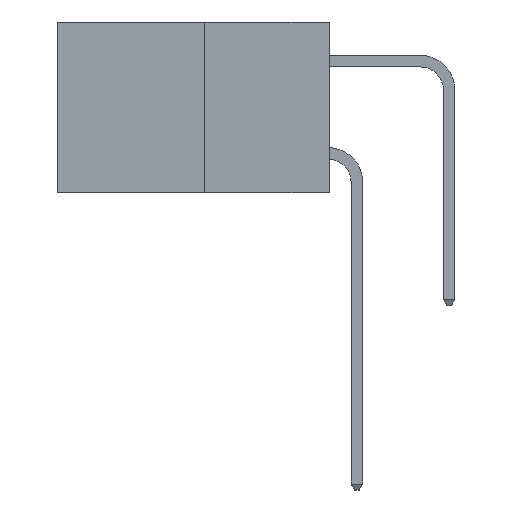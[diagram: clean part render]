
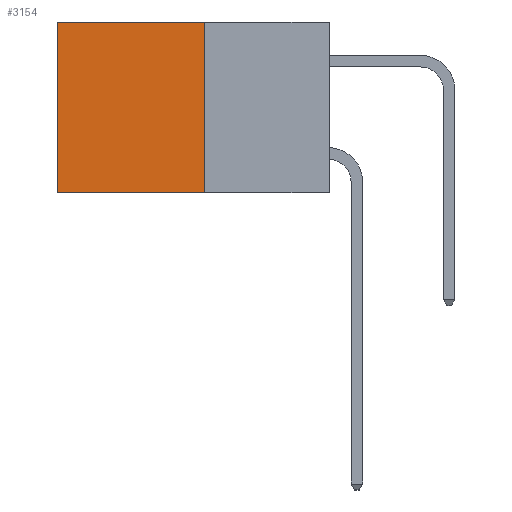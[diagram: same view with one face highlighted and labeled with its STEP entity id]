
A CAD part, left-side view. The second image highlights one B-rep face of the part: STEP entity #3154.
In plain terms, the highlighted planar face has unit normal (-1, 0, 0).
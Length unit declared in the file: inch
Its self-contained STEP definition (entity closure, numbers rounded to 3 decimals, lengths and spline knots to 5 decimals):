
#907 = EDGE_CURVE ( 'NONE', #5176, #29752, #3105, .T. ) ;
#1414 = EDGE_LOOP ( 'NONE', ( #25171, #21873, #22550, #12734 ) ) ;
#3019 = CARTESIAN_POINT ( 'NONE',  ( 0.277, 0.27, -0.37 ) ) ;
#3105 = LINE ( 'NONE', #26412, #15734 ) ;
#3154 = ADVANCED_FACE ( 'NONE', ( #15588 ), #24416, .F. ) ;
#4847 = VERTEX_POINT ( 'NONE', #13931 ) ;
#5176 = VERTEX_POINT ( 'NONE', #19872 ) ;
#7622 = VERTEX_POINT ( 'NONE', #25596 ) ;
#8562 = VECTOR ( 'NONE', #15060, 39.37008 ) ;
#9820 = DIRECTION ( 'NONE',  ( 0., 1., 0. ) ) ;
#10041 = DIRECTION ( 'NONE',  ( 1., 0., 0. ) ) ;
#10617 = DIRECTION ( 'NONE',  ( 0., 0., -1. ) ) ;
#11900 = CARTESIAN_POINT ( 'NONE',  ( 0.277, 0.27, 0. ) ) ;
#12734 = ORIENTED_EDGE ( 'NONE', *, *, #28041, .T. ) ;
#13288 = VECTOR ( 'NONE', #9820, 39.37008 ) ;
#13931 = CARTESIAN_POINT ( 'NONE',  ( 0.277, 0.27, -0.37 ) ) ;
#14045 = LINE ( 'NONE', #19336, #13288 ) ;
#14909 = LINE ( 'NONE', #3019, #8562 ) ;
#15060 = DIRECTION ( 'NONE',  ( 0., 0., -1. ) ) ;
#15588 = FACE_OUTER_BOUND ( 'NONE', #1414, .T. ) ;
#15734 = VECTOR ( 'NONE', #10617, 39.37008 ) ;
#19024 = AXIS2_PLACEMENT_3D ( 'NONE', #19559, #10041, #26860 ) ;
#19336 = CARTESIAN_POINT ( 'NONE',  ( 0.277, 0.27, -0.37 ) ) ;
#19559 = CARTESIAN_POINT ( 'NONE',  ( 0.277, 0.27, -0.37 ) ) ;
#19872 = CARTESIAN_POINT ( 'NONE',  ( 0.277, 0.59, 0. ) ) ;
#21571 = DIRECTION ( 'NONE',  ( 0., 1., 0. ) ) ;
#21873 = ORIENTED_EDGE ( 'NONE', *, *, #28126, .F. ) ;
#21943 = VECTOR ( 'NONE', #21571, 39.37008 ) ;
#22550 = ORIENTED_EDGE ( 'NONE', *, *, #23239, .F. ) ;
#23239 = EDGE_CURVE ( 'NONE', #7622, #4847, #14909, .T. ) ;
#24416 = PLANE ( 'NONE',  #19024 ) ;
#25171 = ORIENTED_EDGE ( 'NONE', *, *, #907, .T. ) ;
#25596 = CARTESIAN_POINT ( 'NONE',  ( 0.277, 0.27, 0. ) ) ;
#26412 = CARTESIAN_POINT ( 'NONE',  ( 0.277, 0.59, -0.37 ) ) ;
#26860 = DIRECTION ( 'NONE',  ( 0., 0., -1. ) ) ;
#28041 = EDGE_CURVE ( 'NONE', #7622, #5176, #28336, .T. ) ;
#28126 = EDGE_CURVE ( 'NONE', #4847, #29752, #14045, .T. ) ;
#28148 = CARTESIAN_POINT ( 'NONE',  ( 0.277, 0.59, -0.37 ) ) ;
#28336 = LINE ( 'NONE', #11900, #21943 ) ;
#29752 = VERTEX_POINT ( 'NONE', #28148 ) ;
